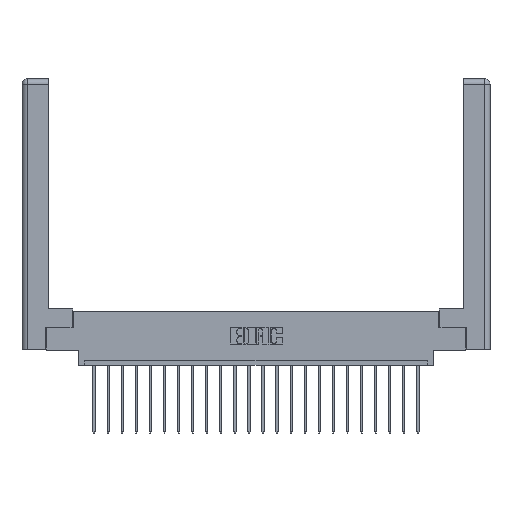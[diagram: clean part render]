
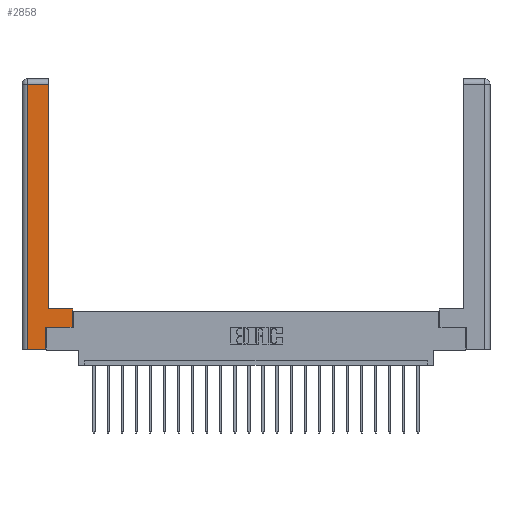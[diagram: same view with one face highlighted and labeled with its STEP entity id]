
A CAD part, top view. The second image highlights one B-rep face of the part: STEP entity #2858.
In plain terms, the highlighted planar face has unit normal (0, 0, 1).
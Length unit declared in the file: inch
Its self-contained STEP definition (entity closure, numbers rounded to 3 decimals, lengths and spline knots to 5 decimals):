
#102 = VECTOR ( 'NONE', #22150, 39.37008 ) ;
#520 = EDGE_CURVE ( 'NONE', #13714, #1583, #5348, .T. ) ;
#610 = DIRECTION ( 'NONE',  ( 0., 1., 0. ) ) ;
#833 = CARTESIAN_POINT ( 'NONE',  ( 0.295, 2.94, 0. ) ) ;
#936 = CARTESIAN_POINT ( 'NONE',  ( 0.265, 0., 0. ) ) ;
#1583 = VERTEX_POINT ( 'NONE', #4949 ) ;
#1587 = VECTOR ( 'NONE', #2424, 39.37008 ) ;
#1661 = VECTOR ( 'NONE', #13704, 39.37008 ) ;
#2152 = AXIS2_PLACEMENT_3D ( 'NONE', #16638, #5977, #22085 ) ;
#2424 = DIRECTION ( 'NONE',  ( 0., -1., 0. ) ) ;
#2670 = DIRECTION ( 'NONE',  ( 1., 0., 0. ) ) ;
#2858 = ADVANCED_FACE ( 'NONE', ( #11420 ), #18494, .F. ) ;
#2881 = LINE ( 'NONE', #13197, #3424 ) ;
#2980 = CARTESIAN_POINT ( 'NONE',  ( 0.265, 0., 0. ) ) ;
#3043 = LINE ( 'NONE', #10392, #13586 ) ;
#3424 = VECTOR ( 'NONE', #19958, 39.37008 ) ;
#3437 = LINE ( 'NONE', #936, #19253 ) ;
#4356 = CARTESIAN_POINT ( 'NONE',  ( 0.0615, 0., 0. ) ) ;
#4891 = VERTEX_POINT ( 'NONE', #13392 ) ;
#4949 = CARTESIAN_POINT ( 'NONE',  ( 0.0615, 2.94, 0. ) ) ;
#5021 = CARTESIAN_POINT ( 'NONE',  ( 0.265, 0.245, 0. ) ) ;
#5348 = LINE ( 'NONE', #18333, #102 ) ;
#5380 = CARTESIAN_POINT ( 'NONE',  ( 0.565, 0.245, 0. ) ) ;
#5706 = CARTESIAN_POINT ( 'NONE',  ( 0.295, 0.45, 0. ) ) ;
#5977 = DIRECTION ( 'NONE',  ( 0., 0., -1. ) ) ;
#6366 = ORIENTED_EDGE ( 'NONE', *, *, #16443, .T. ) ;
#6473 = EDGE_CURVE ( 'NONE', #18569, #13262, #3437, .T. ) ;
#7309 = ORIENTED_EDGE ( 'NONE', *, *, #21114, .T. ) ;
#7715 = DIRECTION ( 'NONE',  ( 1., 0., 0. ) ) ;
#8603 = ORIENTED_EDGE ( 'NONE', *, *, #15946, .T. ) ;
#9056 = EDGE_CURVE ( 'NONE', #1583, #18569, #18483, .T. ) ;
#9420 = CARTESIAN_POINT ( 'NONE',  ( 0.565, 0.245, 0. ) ) ;
#10392 = CARTESIAN_POINT ( 'NONE',  ( 0.295, 3., 0. ) ) ;
#11420 = FACE_OUTER_BOUND ( 'NONE', #16938, .T. ) ;
#11447 = ORIENTED_EDGE ( 'NONE', *, *, #6473, .T. ) ;
#12756 = ORIENTED_EDGE ( 'NONE', *, *, #22340, .T. ) ;
#13197 = CARTESIAN_POINT ( 'NONE',  ( 0.295, 0.45, 0. ) ) ;
#13262 = VERTEX_POINT ( 'NONE', #2980 ) ;
#13392 = CARTESIAN_POINT ( 'NONE',  ( 0.265, 0.245, 0. ) ) ;
#13586 = VECTOR ( 'NONE', #22829, 39.37008 ) ;
#13704 = DIRECTION ( 'NONE',  ( 0., 1., 0. ) ) ;
#13714 = VERTEX_POINT ( 'NONE', #833 ) ;
#13894 = LINE ( 'NONE', #5021, #1661 ) ;
#14287 = VECTOR ( 'NONE', #7715, 39.37008 ) ;
#14344 = VERTEX_POINT ( 'NONE', #5706 ) ;
#15539 = ORIENTED_EDGE ( 'NONE', *, *, #9056, .T. ) ;
#15642 = CARTESIAN_POINT ( 'NONE',  ( 0.565, 0.45, 0. ) ) ;
#15946 = EDGE_CURVE ( 'NONE', #13262, #4891, #13894, .T. ) ;
#16266 = VERTEX_POINT ( 'NONE', #15642 ) ;
#16341 = ORIENTED_EDGE ( 'NONE', *, *, #22359, .T. ) ;
#16443 = EDGE_CURVE ( 'NONE', #14344, #13714, #3043, .T. ) ;
#16638 = CARTESIAN_POINT ( 'NONE',  ( 0., 0., 0. ) ) ;
#16938 = EDGE_LOOP ( 'NONE', ( #6366, #17734, #15539, #11447, #8603, #7309, #16341, #12756 ) ) ;
#16998 = VECTOR ( 'NONE', #610, 39.37008 ) ;
#17543 = LINE ( 'NONE', #21821, #16998 ) ;
#17734 = ORIENTED_EDGE ( 'NONE', *, *, #520, .T. ) ;
#18333 = CARTESIAN_POINT ( 'NONE',  ( 0.0615, 2.94, 0. ) ) ;
#18483 = LINE ( 'NONE', #20674, #1587 ) ;
#18494 = PLANE ( 'NONE',  #2152 ) ;
#18569 = VERTEX_POINT ( 'NONE', #4356 ) ;
#19007 = LINE ( 'NONE', #9420, #14287 ) ;
#19253 = VECTOR ( 'NONE', #2670, 39.37008 ) ;
#19958 = DIRECTION ( 'NONE',  ( -1., 0., 0. ) ) ;
#20674 = CARTESIAN_POINT ( 'NONE',  ( 0.0615, 0., 0. ) ) ;
#21114 = EDGE_CURVE ( 'NONE', #4891, #21763, #19007, .T. ) ;
#21763 = VERTEX_POINT ( 'NONE', #5380 ) ;
#21821 = CARTESIAN_POINT ( 'NONE',  ( 0.565, 0.45, 0. ) ) ;
#22085 = DIRECTION ( 'NONE',  ( -1., 0., 0. ) ) ;
#22150 = DIRECTION ( 'NONE',  ( -1., 0., 0. ) ) ;
#22340 = EDGE_CURVE ( 'NONE', #16266, #14344, #2881, .T. ) ;
#22359 = EDGE_CURVE ( 'NONE', #21763, #16266, #17543, .T. ) ;
#22829 = DIRECTION ( 'NONE',  ( 0., 1., 0. ) ) ;
